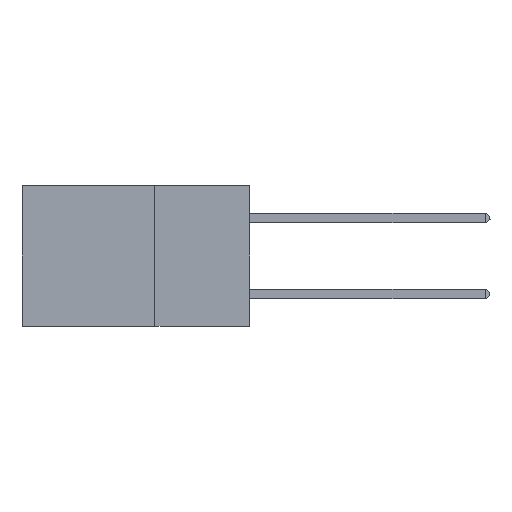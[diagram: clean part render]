
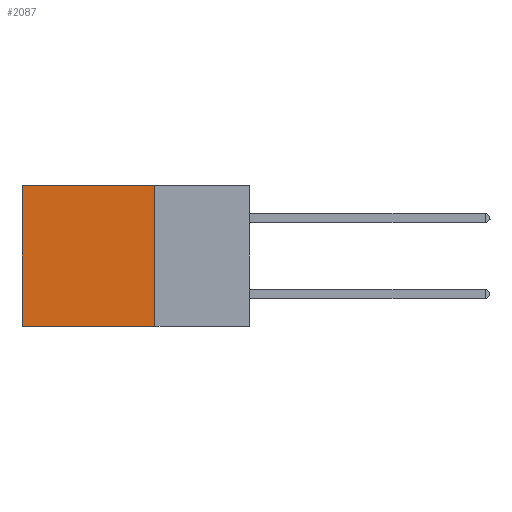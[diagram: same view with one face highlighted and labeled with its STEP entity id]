
A CAD part, left-side view. The second image highlights one B-rep face of the part: STEP entity #2087.
In plain terms, the highlighted planar face has unit normal (-1, 0, 0).
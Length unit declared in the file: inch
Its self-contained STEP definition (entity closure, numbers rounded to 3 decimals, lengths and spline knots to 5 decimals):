
#277 = VECTOR ( 'NONE', #22831, 39.37008 ) ;
#636 = EDGE_LOOP ( 'NONE', ( #3243, #3329, #29172, #23937 ) ) ;
#1288 = CARTESIAN_POINT ( 'NONE',  ( 0.2875, 0.25, 0. ) ) ;
#2087 = ADVANCED_FACE ( 'NONE', ( #33093 ), #33260, .F. ) ;
#2675 = VERTEX_POINT ( 'NONE', #21422 ) ;
#3243 = ORIENTED_EDGE ( 'NONE', *, *, #21110, .T. ) ;
#3329 = ORIENTED_EDGE ( 'NONE', *, *, #9120, .F. ) ;
#4758 = CARTESIAN_POINT ( 'NONE',  ( 0.2875, 0.25, -0.37 ) ) ;
#4760 = CARTESIAN_POINT ( 'NONE',  ( 0.2875, 0.25, 0. ) ) ;
#7288 = VECTOR ( 'NONE', #33179, 39.37008 ) ;
#8843 = CARTESIAN_POINT ( 'NONE',  ( 0.2875, 0.25, -0.37 ) ) ;
#8936 = LINE ( 'NONE', #16510, #19436 ) ;
#9120 = EDGE_CURVE ( 'NONE', #10877, #28182, #11919, .T. ) ;
#10877 = VERTEX_POINT ( 'NONE', #4758 ) ;
#11136 = EDGE_CURVE ( 'NONE', #32974, #10877, #17144, .T. ) ;
#11919 = LINE ( 'NONE', #8843, #23126 ) ;
#12527 = EDGE_CURVE ( 'NONE', #32974, #2675, #8936, .T. ) ;
#16510 = CARTESIAN_POINT ( 'NONE',  ( 0.2875, 0.25, 0. ) ) ;
#17144 = LINE ( 'NONE', #1288, #7288 ) ;
#17224 = DIRECTION ( 'NONE',  ( 1., 0., 0. ) ) ;
#17500 = LINE ( 'NONE', #28013, #277 ) ;
#19436 = VECTOR ( 'NONE', #27196, 39.37008 ) ;
#21110 = EDGE_CURVE ( 'NONE', #2675, #28182, #17500, .T. ) ;
#21422 = CARTESIAN_POINT ( 'NONE',  ( 0.2875, 0.6, 0. ) ) ;
#22831 = DIRECTION ( 'NONE',  ( 0., 0., -1. ) ) ;
#23126 = VECTOR ( 'NONE', #30189, 39.37008 ) ;
#23937 = ORIENTED_EDGE ( 'NONE', *, *, #12527, .T. ) ;
#25320 = DIRECTION ( 'NONE',  ( 0., 0., -1. ) ) ;
#27196 = DIRECTION ( 'NONE',  ( 0., 1., 0. ) ) ;
#27675 = AXIS2_PLACEMENT_3D ( 'NONE', #30329, #17224, #25320 ) ;
#28013 = CARTESIAN_POINT ( 'NONE',  ( 0.2875, 0.6, 0. ) ) ;
#28182 = VERTEX_POINT ( 'NONE', #31256 ) ;
#29172 = ORIENTED_EDGE ( 'NONE', *, *, #11136, .F. ) ;
#30189 = DIRECTION ( 'NONE',  ( 0., 1., 0. ) ) ;
#30329 = CARTESIAN_POINT ( 'NONE',  ( 0.2875, 0.25, 0. ) ) ;
#31256 = CARTESIAN_POINT ( 'NONE',  ( 0.2875, 0.6, -0.37 ) ) ;
#32974 = VERTEX_POINT ( 'NONE', #4760 ) ;
#33093 = FACE_OUTER_BOUND ( 'NONE', #636, .T. ) ;
#33179 = DIRECTION ( 'NONE',  ( 0., 0., -1. ) ) ;
#33260 = PLANE ( 'NONE',  #27675 ) ;
